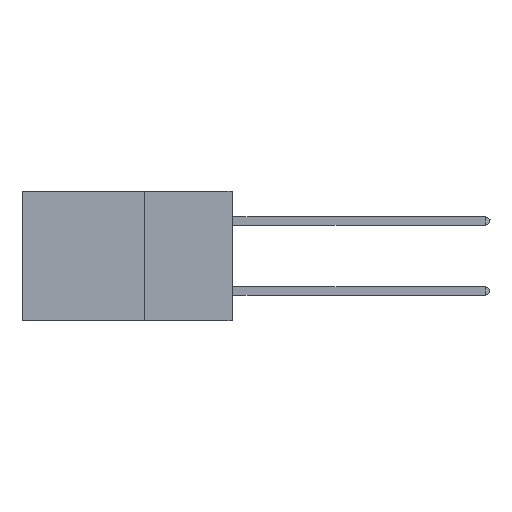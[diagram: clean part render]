
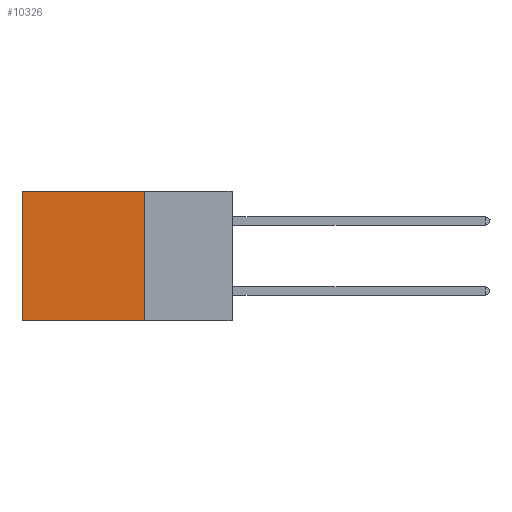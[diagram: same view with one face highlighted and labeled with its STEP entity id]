
A CAD part, left-side view. The second image highlights one B-rep face of the part: STEP entity #10326.
In plain terms, the highlighted planar face has unit normal (-1, 0, 0).
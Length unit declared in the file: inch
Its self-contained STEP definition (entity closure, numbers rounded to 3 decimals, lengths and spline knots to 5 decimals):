
#520 = CARTESIAN_POINT ( 'NONE',  ( 0.2875, 0.6, -0.37 ) ) ;
#650 = ORIENTED_EDGE ( 'NONE', *, *, #7893, .F. ) ;
#1390 = PLANE ( 'NONE',  #15126 ) ;
#2875 = FACE_OUTER_BOUND ( 'NONE', #9721, .T. ) ;
#3301 = ORIENTED_EDGE ( 'NONE', *, *, #9109, .T. ) ;
#3680 = CARTESIAN_POINT ( 'NONE',  ( 0.2875, 0.25, 0. ) ) ;
#3878 = VERTEX_POINT ( 'NONE', #4229 ) ;
#4229 = CARTESIAN_POINT ( 'NONE',  ( 0.2875, 0.6, 0. ) ) ;
#4322 = ORIENTED_EDGE ( 'NONE', *, *, #16096, .T. ) ;
#4350 = CARTESIAN_POINT ( 'NONE',  ( 0.2875, 0.6, 0. ) ) ;
#4585 = LINE ( 'NONE', #4350, #10363 ) ;
#5214 = VECTOR ( 'NONE', #13748, 39.37008 ) ;
#5309 = VERTEX_POINT ( 'NONE', #520 ) ;
#5344 = DIRECTION ( 'NONE',  ( 0., 0., -1. ) ) ;
#7023 = LINE ( 'NONE', #11990, #12794 ) ;
#7684 = LINE ( 'NONE', #13889, #10630 ) ;
#7893 = EDGE_CURVE ( 'NONE', #10683, #5309, #7684, .T. ) ;
#8975 = CARTESIAN_POINT ( 'NONE',  ( 0.2875, 0.25, 0. ) ) ;
#9109 = EDGE_CURVE ( 'NONE', #3878, #5309, #4585, .T. ) ;
#9218 = DIRECTION ( 'NONE',  ( 1., 0., 0. ) ) ;
#9514 = DIRECTION ( 'NONE',  ( 0., 0., -1. ) ) ;
#9721 = EDGE_LOOP ( 'NONE', ( #3301, #650, #14123, #4322 ) ) ;
#9929 = CARTESIAN_POINT ( 'NONE',  ( 0.2875, 0.25, 0. ) ) ;
#10006 = DIRECTION ( 'NONE',  ( 0., 1., 0. ) ) ;
#10326 = ADVANCED_FACE ( 'NONE', ( #2875 ), #1390, .F. ) ;
#10363 = VECTOR ( 'NONE', #15659, 39.37008 ) ;
#10630 = VECTOR ( 'NONE', #10006, 39.37008 ) ;
#10683 = VERTEX_POINT ( 'NONE', #11342 ) ;
#10987 = EDGE_CURVE ( 'NONE', #11108, #10683, #7023, .T. ) ;
#11108 = VERTEX_POINT ( 'NONE', #9929 ) ;
#11342 = CARTESIAN_POINT ( 'NONE',  ( 0.2875, 0.25, -0.37 ) ) ;
#11516 = LINE ( 'NONE', #3680, #5214 ) ;
#11990 = CARTESIAN_POINT ( 'NONE',  ( 0.2875, 0.25, 0. ) ) ;
#12794 = VECTOR ( 'NONE', #9514, 39.37008 ) ;
#13748 = DIRECTION ( 'NONE',  ( 0., 1., 0. ) ) ;
#13889 = CARTESIAN_POINT ( 'NONE',  ( 0.2875, 0.25, -0.37 ) ) ;
#14123 = ORIENTED_EDGE ( 'NONE', *, *, #10987, .F. ) ;
#15126 = AXIS2_PLACEMENT_3D ( 'NONE', #8975, #9218, #5344 ) ;
#15659 = DIRECTION ( 'NONE',  ( 0., 0., -1. ) ) ;
#16096 = EDGE_CURVE ( 'NONE', #11108, #3878, #11516, .T. ) ;
